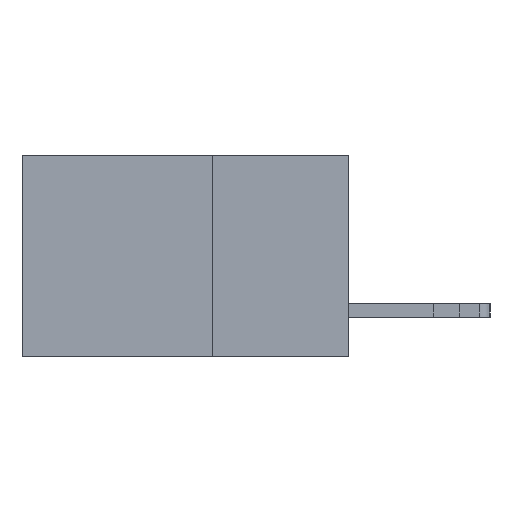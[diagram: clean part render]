
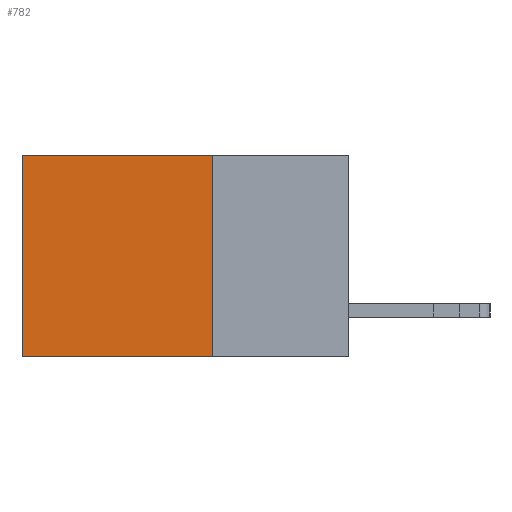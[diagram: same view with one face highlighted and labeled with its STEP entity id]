
A CAD part, left-side view. The second image highlights one B-rep face of the part: STEP entity #782.
In plain terms, the highlighted planar face has unit normal (-1, 0, 0).
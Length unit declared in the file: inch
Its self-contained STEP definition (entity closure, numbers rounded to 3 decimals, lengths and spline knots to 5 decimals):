
#520 = VECTOR ( 'NONE', #9628, 39.37008 ) ;
#753 = DIRECTION ( 'NONE',  ( 1., 0., 0. ) ) ;
#782 = ADVANCED_FACE ( 'NONE', ( #13233 ), #8260, .F. ) ;
#913 = LINE ( 'NONE', #8409, #520 ) ;
#1019 = VECTOR ( 'NONE', #10291, 39.37008 ) ;
#1575 = ORIENTED_EDGE ( 'NONE', *, *, #10077, .F. ) ;
#2030 = ORIENTED_EDGE ( 'NONE', *, *, #14354, .F. ) ;
#2479 = DIRECTION ( 'NONE',  ( 0., 1., 0. ) ) ;
#3153 = VECTOR ( 'NONE', #2479, 39.37008 ) ;
#3204 = CARTESIAN_POINT ( 'NONE',  ( 0.298, 0.25, 0. ) ) ;
#3269 = ORIENTED_EDGE ( 'NONE', *, *, #8287, .T. ) ;
#3413 = DIRECTION ( 'NONE',  ( 0., 0., -1. ) ) ;
#3460 = VERTEX_POINT ( 'NONE', #4498 ) ;
#3529 = CARTESIAN_POINT ( 'NONE',  ( 0.298, 0.25, 0. ) ) ;
#4498 = CARTESIAN_POINT ( 'NONE',  ( 0.298, 0.6, -0.37 ) ) ;
#4807 = CARTESIAN_POINT ( 'NONE',  ( 0.298, 0.6, 0. ) ) ;
#4854 = DIRECTION ( 'NONE',  ( 0., 0., -1. ) ) ;
#5005 = CARTESIAN_POINT ( 'NONE',  ( 0.298, 0.25, -0.37 ) ) ;
#6415 = LINE ( 'NONE', #5005, #3153 ) ;
#6971 = CARTESIAN_POINT ( 'NONE',  ( 0.298, 0.25, -0.37 ) ) ;
#7423 = EDGE_CURVE ( 'NONE', #8968, #14468, #7958, .T. ) ;
#7484 = VERTEX_POINT ( 'NONE', #6971 ) ;
#7929 = VECTOR ( 'NONE', #4854, 39.37008 ) ;
#7958 = LINE ( 'NONE', #3204, #1019 ) ;
#8260 = PLANE ( 'NONE',  #11651 ) ;
#8287 = EDGE_CURVE ( 'NONE', #14468, #3460, #14208, .T. ) ;
#8409 = CARTESIAN_POINT ( 'NONE',  ( 0.298, 0.25, 0. ) ) ;
#8479 = CARTESIAN_POINT ( 'NONE',  ( 0.298, 0.25, 0. ) ) ;
#8968 = VERTEX_POINT ( 'NONE', #3529 ) ;
#9628 = DIRECTION ( 'NONE',  ( 0., 0., -1. ) ) ;
#9811 = CARTESIAN_POINT ( 'NONE',  ( 0.298, 0.6, 0. ) ) ;
#10077 = EDGE_CURVE ( 'NONE', #7484, #3460, #6415, .T. ) ;
#10291 = DIRECTION ( 'NONE',  ( 0., 1., 0. ) ) ;
#10516 = EDGE_LOOP ( 'NONE', ( #3269, #1575, #2030, #11924 ) ) ;
#11651 = AXIS2_PLACEMENT_3D ( 'NONE', #8479, #753, #3413 ) ;
#11924 = ORIENTED_EDGE ( 'NONE', *, *, #7423, .T. ) ;
#13233 = FACE_OUTER_BOUND ( 'NONE', #10516, .T. ) ;
#14208 = LINE ( 'NONE', #4807, #7929 ) ;
#14354 = EDGE_CURVE ( 'NONE', #8968, #7484, #913, .T. ) ;
#14468 = VERTEX_POINT ( 'NONE', #9811 ) ;
